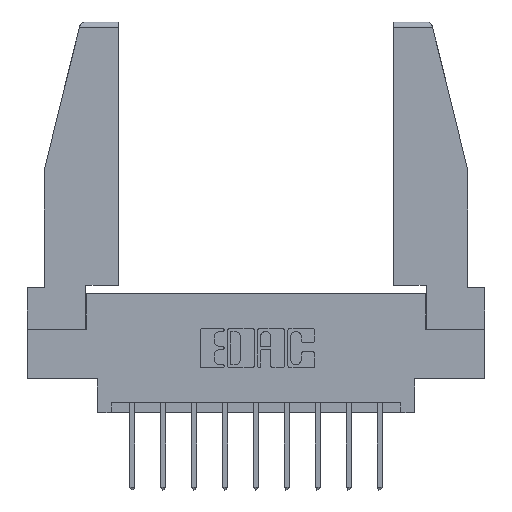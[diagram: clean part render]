
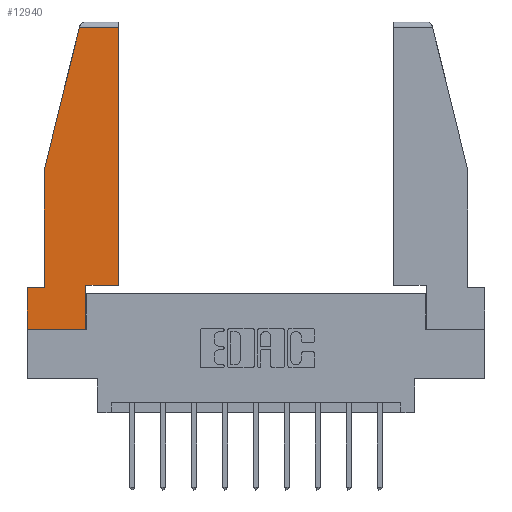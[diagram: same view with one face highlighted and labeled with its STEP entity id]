
A CAD part, top view. The second image highlights one B-rep face of the part: STEP entity #12940.
In plain terms, the highlighted planar face has unit normal (0, 0, 1).
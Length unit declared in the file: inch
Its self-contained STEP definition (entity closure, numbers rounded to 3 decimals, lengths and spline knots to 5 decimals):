
#253 = LINE ( 'NONE', #12473, #11371 ) ;
#412 = LINE ( 'NONE', #11029, #4607 ) ;
#437 = CARTESIAN_POINT ( 'NONE',  ( 0.297, 0., 0. ) ) ;
#544 = VECTOR ( 'NONE', #7863, 39.37008 ) ;
#648 = VERTEX_POINT ( 'NONE', #10381 ) ;
#655 = EDGE_CURVE ( 'NONE', #2692, #9412, #253, .T. ) ;
#946 = DIRECTION ( 'NONE',  ( 0., -1., 0. ) ) ;
#1100 = EDGE_CURVE ( 'NONE', #12093, #4166, #412, .T. ) ;
#1409 = DIRECTION ( 'NONE',  ( 1., 0., 0. ) ) ;
#1416 = CARTESIAN_POINT ( 'NONE',  ( 0.2636, 1.52, 0. ) ) ;
#1654 = VERTEX_POINT ( 'NONE', #437 ) ;
#1726 = VERTEX_POINT ( 'NONE', #4850 ) ;
#2074 = CARTESIAN_POINT ( 'NONE',  ( 0., 0.21, 0. ) ) ;
#2143 = EDGE_CURVE ( 'NONE', #648, #1726, #5779, .T. ) ;
#2183 = CARTESIAN_POINT ( 'NONE',  ( 0.461, 0.223, 0. ) ) ;
#2692 = VERTEX_POINT ( 'NONE', #2074 ) ;
#3078 = LINE ( 'NONE', #2183, #6737 ) ;
#3230 = ORIENTED_EDGE ( 'NONE', *, *, #655, .T. ) ;
#3372 = VECTOR ( 'NONE', #7365, 39.37008 ) ;
#3428 = DIRECTION ( 'NONE',  ( 1., 0., 0. ) ) ;
#4013 = ORIENTED_EDGE ( 'NONE', *, *, #2143, .T. ) ;
#4166 = VERTEX_POINT ( 'NONE', #6814 ) ;
#4305 = AXIS2_PLACEMENT_3D ( 'NONE', #5353, #12865, #3428 ) ;
#4480 = ORIENTED_EDGE ( 'NONE', *, *, #10319, .T. ) ;
#4607 = VECTOR ( 'NONE', #1409, 39.37008 ) ;
#4787 = VERTEX_POINT ( 'NONE', #1416 ) ;
#4850 = CARTESIAN_POINT ( 'NONE',  ( 0.086, 0.21, 0. ) ) ;
#4864 = CARTESIAN_POINT ( 'NONE',  ( 0.271, 1.55, 0. ) ) ;
#4993 = CARTESIAN_POINT ( 'NONE',  ( 0., 1.52, 0. ) ) ;
#5238 = VERTEX_POINT ( 'NONE', #6808 ) ;
#5353 = CARTESIAN_POINT ( 'NONE',  ( 0., 0., 0. ) ) ;
#5376 = LINE ( 'NONE', #9621, #6516 ) ;
#5464 = EDGE_CURVE ( 'NONE', #5238, #4787, #12840, .T. ) ;
#5543 = EDGE_CURVE ( 'NONE', #4166, #5238, #3078, .T. ) ;
#5753 = DIRECTION ( 'NONE',  ( 1., 0., 0. ) ) ;
#5779 = LINE ( 'NONE', #10706, #10627 ) ;
#5787 = EDGE_LOOP ( 'NONE', ( #11905, #5797, #4480, #4013, #10356, #3230, #6378, #7792, #10103 ) ) ;
#5797 = ORIENTED_EDGE ( 'NONE', *, *, #5464, .T. ) ;
#6194 = LINE ( 'NONE', #8374, #3372 ) ;
#6378 = ORIENTED_EDGE ( 'NONE', *, *, #11926, .T. ) ;
#6411 = PLANE ( 'NONE',  #4305 ) ;
#6516 = VECTOR ( 'NONE', #10809, 39.37008 ) ;
#6737 = VECTOR ( 'NONE', #13847, 39.37008 ) ;
#6808 = CARTESIAN_POINT ( 'NONE',  ( 0.461, 1.52, 0. ) ) ;
#6814 = CARTESIAN_POINT ( 'NONE',  ( 0.461, 0.223, 0. ) ) ;
#7034 = LINE ( 'NONE', #7831, #9394 ) ;
#7365 = DIRECTION ( 'NONE',  ( -1., 0., 0. ) ) ;
#7792 = ORIENTED_EDGE ( 'NONE', *, *, #12586, .T. ) ;
#7831 = CARTESIAN_POINT ( 'NONE',  ( 0., 0., 0. ) ) ;
#7863 = DIRECTION ( 'NONE',  ( -0.239, -0.971, 0. ) ) ;
#8374 = CARTESIAN_POINT ( 'NONE',  ( 0., 0.21, 0. ) ) ;
#9361 = CARTESIAN_POINT ( 'NONE',  ( 0.297, 0.223, 0. ) ) ;
#9394 = VECTOR ( 'NONE', #5753, 39.37008 ) ;
#9412 = VERTEX_POINT ( 'NONE', #13801 ) ;
#9621 = CARTESIAN_POINT ( 'NONE',  ( 0.297, 0., 0. ) ) ;
#9956 = VECTOR ( 'NONE', #12483, 39.37008 ) ;
#10103 = ORIENTED_EDGE ( 'NONE', *, *, #1100, .T. ) ;
#10319 = EDGE_CURVE ( 'NONE', #4787, #648, #10578, .T. ) ;
#10337 = DIRECTION ( 'NONE',  ( 0., -1., 0. ) ) ;
#10356 = ORIENTED_EDGE ( 'NONE', *, *, #12489, .T. ) ;
#10381 = CARTESIAN_POINT ( 'NONE',  ( 0.086, 0.8, 0. ) ) ;
#10578 = LINE ( 'NONE', #4864, #544 ) ;
#10627 = VECTOR ( 'NONE', #946, 39.37008 ) ;
#10706 = CARTESIAN_POINT ( 'NONE',  ( 0.086, 0.8, 0. ) ) ;
#10809 = DIRECTION ( 'NONE',  ( 0., 1., 0. ) ) ;
#11029 = CARTESIAN_POINT ( 'NONE',  ( 0.297, 0.223, 0. ) ) ;
#11371 = VECTOR ( 'NONE', #10337, 39.37008 ) ;
#11905 = ORIENTED_EDGE ( 'NONE', *, *, #5543, .T. ) ;
#11926 = EDGE_CURVE ( 'NONE', #9412, #1654, #7034, .T. ) ;
#12093 = VERTEX_POINT ( 'NONE', #9361 ) ;
#12473 = CARTESIAN_POINT ( 'NONE',  ( 0., 0.21, 0. ) ) ;
#12483 = DIRECTION ( 'NONE',  ( -1., 0., 0. ) ) ;
#12489 = EDGE_CURVE ( 'NONE', #1726, #2692, #6194, .T. ) ;
#12586 = EDGE_CURVE ( 'NONE', #1654, #12093, #5376, .T. ) ;
#12840 = LINE ( 'NONE', #4993, #9956 ) ;
#12865 = DIRECTION ( 'NONE',  ( 0., 0., 1. ) ) ;
#12940 = ADVANCED_FACE ( 'NONE', ( #13090 ), #6411, .T. ) ;
#13090 = FACE_OUTER_BOUND ( 'NONE', #5787, .T. ) ;
#13801 = CARTESIAN_POINT ( 'NONE',  ( 0., 0., 0. ) ) ;
#13847 = DIRECTION ( 'NONE',  ( 0., 1., 0. ) ) ;
